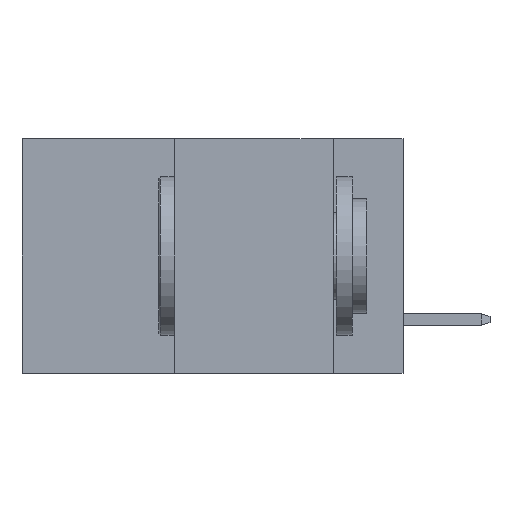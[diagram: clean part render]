
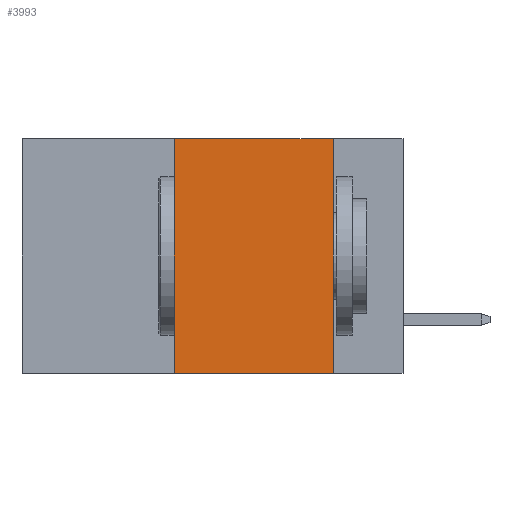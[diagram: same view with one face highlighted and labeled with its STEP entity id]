
A CAD part, left-side view. The second image highlights one B-rep face of the part: STEP entity #3993.
In plain terms, the highlighted planar face has unit normal (-1, 0, 0).
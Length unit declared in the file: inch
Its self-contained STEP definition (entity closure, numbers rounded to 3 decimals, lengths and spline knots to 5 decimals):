
#1618 = LINE ( 'NONE', #1784, #20564 ) ;
#1784 = CARTESIAN_POINT ( 'NONE',  ( 0., 0.11, 0. ) ) ;
#2571 = FACE_OUTER_BOUND ( 'NONE', #2696, .T. ) ;
#2696 = EDGE_LOOP ( 'NONE', ( #8944, #26341, #6204, #4414 ) ) ;
#2782 = VERTEX_POINT ( 'NONE', #22376 ) ;
#3075 = LINE ( 'NONE', #29991, #4197 ) ;
#3993 = ADVANCED_FACE ( 'NONE', ( #2571 ), #19978, .F. ) ;
#4197 = VECTOR ( 'NONE', #15648, 39.37008 ) ;
#4414 = ORIENTED_EDGE ( 'NONE', *, *, #21965, .T. ) ;
#4989 = DIRECTION ( 'NONE',  ( 0., 0., 1. ) ) ;
#5009 = CARTESIAN_POINT ( 'NONE',  ( 0., 0.6, 0. ) ) ;
#6204 = ORIENTED_EDGE ( 'NONE', *, *, #28067, .F. ) ;
#7800 = VERTEX_POINT ( 'NONE', #15796 ) ;
#8609 = EDGE_CURVE ( 'NONE', #14877, #7800, #3075, .T. ) ;
#8944 = ORIENTED_EDGE ( 'NONE', *, *, #18719, .F. ) ;
#8999 = DIRECTION ( 'NONE',  ( 0., -1., 0. ) ) ;
#9490 = CARTESIAN_POINT ( 'NONE',  ( 0., 0.36, 0. ) ) ;
#11425 = LINE ( 'NONE', #14002, #21517 ) ;
#14002 = CARTESIAN_POINT ( 'NONE',  ( 0., 0.6, -0.37 ) ) ;
#14231 = DIRECTION ( 'NONE',  ( 0., 0., -1. ) ) ;
#14841 = DIRECTION ( 'NONE',  ( 0., 0., -1. ) ) ;
#14877 = VERTEX_POINT ( 'NONE', #31063 ) ;
#15320 = DIRECTION ( 'NONE',  ( 1., 0., 0. ) ) ;
#15648 = DIRECTION ( 'NONE',  ( 0., -1., 0. ) ) ;
#15796 = CARTESIAN_POINT ( 'NONE',  ( 0., 0.11, 0. ) ) ;
#18719 = EDGE_CURVE ( 'NONE', #7800, #27487, #1618, .T. ) ;
#18722 = CARTESIAN_POINT ( 'NONE',  ( 0., 0.11, -0.37 ) ) ;
#19287 = VECTOR ( 'NONE', #4989, 39.37008 ) ;
#19788 = LINE ( 'NONE', #9490, #19287 ) ;
#19978 = PLANE ( 'NONE',  #30046 ) ;
#20564 = VECTOR ( 'NONE', #14231, 39.37008 ) ;
#21517 = VECTOR ( 'NONE', #8999, 39.37008 ) ;
#21965 = EDGE_CURVE ( 'NONE', #2782, #27487, #11425, .T. ) ;
#22376 = CARTESIAN_POINT ( 'NONE',  ( 0., 0.36, -0.37 ) ) ;
#26341 = ORIENTED_EDGE ( 'NONE', *, *, #8609, .F. ) ;
#27487 = VERTEX_POINT ( 'NONE', #18722 ) ;
#28067 = EDGE_CURVE ( 'NONE', #2782, #14877, #19788, .T. ) ;
#29991 = CARTESIAN_POINT ( 'NONE',  ( 0., 0.6, 0. ) ) ;
#30046 = AXIS2_PLACEMENT_3D ( 'NONE', #5009, #15320, #14841 ) ;
#31063 = CARTESIAN_POINT ( 'NONE',  ( 0., 0.36, 0. ) ) ;
